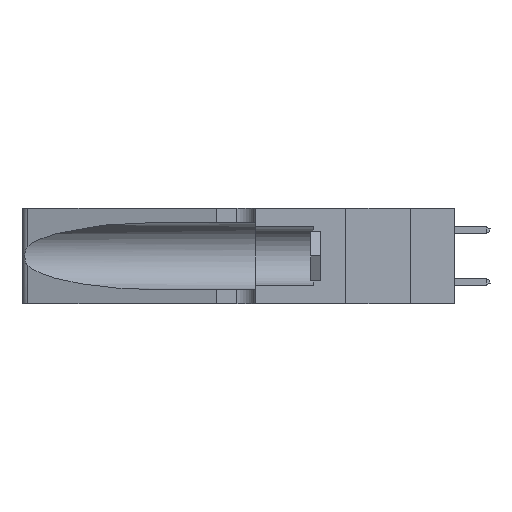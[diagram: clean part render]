
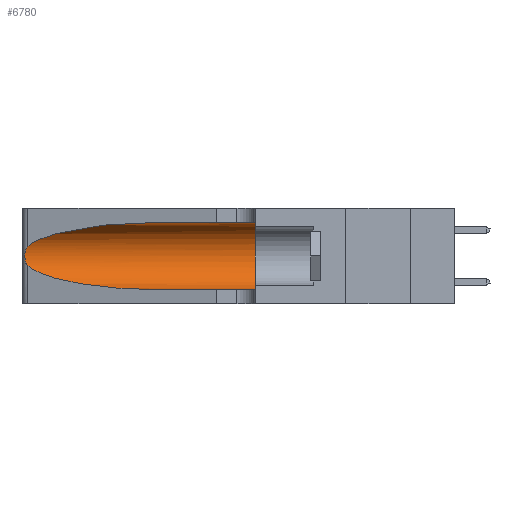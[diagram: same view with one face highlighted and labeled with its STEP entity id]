
A CAD part, left-side view. The second image highlights one B-rep face of the part: STEP entity #6780.
In plain terms, the highlighted cylindrical face has radius 3.308 mm (diameter 6.617 mm), a partial arc.
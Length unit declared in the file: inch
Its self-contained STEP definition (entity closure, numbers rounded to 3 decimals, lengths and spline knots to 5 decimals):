
#3289 = CARTESIAN_POINT ( 'NONE',  ( 0.26075, 1.23896, 0.19203 ) ) ;
#3902 = ORIENTED_EDGE ( 'NONE', *, *, #12680, .F. ) ;
#3939 = CARTESIAN_POINT ( 'NONE',  ( 0.18966, 0.96281, 0.31525 ) ) ;
#4257 = CARTESIAN_POINT ( 'NONE',  ( 0.25487, 1.22718, 0.14631 ) ) ;
#5062 = ORIENTED_EDGE ( 'NONE', *, *, #30417, .T. ) ;
#5416 = DIRECTION ( 'NONE',  ( 0., 1., 0. ) ) ;
#5429 = EDGE_CURVE ( 'NONE', #13423, #27642, #40645, .T. ) ;
#5734 = DIRECTION ( 'NONE',  ( 0., 0., 1. ) ) ;
#6224 = CARTESIAN_POINT ( 'NONE',  ( 0.25487, 1.22718, 0.14631 ) ) ;
#6531 = LINE ( 'NONE', #12979, #15134 ) ;
#6780 = ADVANCED_FACE ( 'NONE', ( #13480 ), #31349, .F. ) ;
#7025 = CARTESIAN_POINT ( 'NONE',  ( 0.25639, 1.23186, 0.15144 ) ) ;
#9495 =( BOUNDED_CURVE ( )  B_SPLINE_CURVE ( 3, ( #40600, #3939, #44308, #36761 ),
 .UNSPECIFIED., .F., .F. ) 
 B_SPLINE_CURVE_WITH_KNOTS ( ( 4, 4 ),
 ( 1.5708, 2.84003 ),
 .UNSPECIFIED. ) 
 CURVE ( )  GEOMETRIC_REPRESENTATION_ITEM ( )  RATIONAL_B_SPLINE_CURVE ( ( 1., 0.87, 0.87, 1. ) ) 
 REPRESENTATION_ITEM ( '' )  );
#10245 = VERTEX_POINT ( 'NONE', #32765 ) ;
#10259 = CARTESIAN_POINT ( 'NONE',  ( 0.25555, 1.22993, 0.14849 ) ) ;
#10776 = AXIS2_PLACEMENT_3D ( 'NONE', #34550, #24108, #42113 ) ;
#12680 = EDGE_CURVE ( 'NONE', #41714, #13423, #20271, .T. ) ;
#12801 = CARTESIAN_POINT ( 'NONE',  ( 0.1305, 0.35, 0.05475 ) ) ;
#12979 = CARTESIAN_POINT ( 'NONE',  ( 0.1305, 1.61858, 0.05475 ) ) ;
#13423 = VERTEX_POINT ( 'NONE', #22677 ) ;
#13480 = FACE_OUTER_BOUND ( 'NONE', #32937, .T. ) ;
#15134 = VECTOR ( 'NONE', #31310, 39.37008 ) ;
#15164 = ORIENTED_EDGE ( 'NONE', *, *, #5429, .F. ) ;
#15608 = AXIS2_PLACEMENT_3D ( 'NONE', #20380, #5416, #5734 ) ;
#15639 = VECTOR ( 'NONE', #41364, 39.37008 ) ;
#17497 = VERTEX_POINT ( 'NONE', #4257 ) ;
#17786 = CARTESIAN_POINT ( 'NONE',  ( 0.26018, 1.23835, 0.19895 ) ) ;
#18111 = CARTESIAN_POINT ( 'NONE',  ( 0.26075, 1.23896, 0.178 ) ) ;
#19822 = ORIENTED_EDGE ( 'NONE', *, *, #21107, .T. ) ;
#20271 = LINE ( 'NONE', #33636, #15639 ) ;
#20380 = CARTESIAN_POINT ( 'NONE',  ( 0.1305, 0.35, 0.185 ) ) ;
#21006 = EDGE_CURVE ( 'NONE', #17497, #45931, #23612, .T. ) ;
#21107 = EDGE_CURVE ( 'NONE', #10245, #17497, #45736, .T. ) ;
#21335 = CARTESIAN_POINT ( 'NONE',  ( 0.26017, 1.23833, 0.17102 ) ) ;
#22677 = CARTESIAN_POINT ( 'NONE',  ( 0.1305, 0.35, 0.31525 ) ) ;
#23612 =( BOUNDED_CURVE ( )  B_SPLINE_CURVE ( 3, ( #6224, #35629, #35780, #24851 ),
 .UNSPECIFIED., .F., .T. ) 
 B_SPLINE_CURVE_WITH_KNOTS ( ( 4, 4 ),
 ( 3.44316, 4.71239 ),
 .UNSPECIFIED. ) 
 CURVE ( )  GEOMETRIC_REPRESENTATION_ITEM ( )  RATIONAL_B_SPLINE_CURVE ( ( 1., 0.87, 0.87, 1. ) ) 
 REPRESENTATION_ITEM ( '' )  );
#24108 = DIRECTION ( 'NONE',  ( 0., -1., 0. ) ) ;
#24851 = CARTESIAN_POINT ( 'NONE',  ( 0.1305, 0.72297, 0.05475 ) ) ;
#25166 = CARTESIAN_POINT ( 'NONE',  ( 0.25787, 1.23484, 0.2124 ) ) ;
#25326 = CARTESIAN_POINT ( 'NONE',  ( 0.25487, 1.22718, 0.22369 ) ) ;
#27642 = VERTEX_POINT ( 'NONE', #12801 ) ;
#28156 = CARTESIAN_POINT ( 'NONE',  ( 0.1305, 0.72297, 0.05475 ) ) ;
#28545 = CARTESIAN_POINT ( 'NONE',  ( 0.25856, 1.23593, 0.16098 ) ) ;
#29025 = CARTESIAN_POINT ( 'NONE',  ( 0.25854, 1.2359, 0.20912 ) ) ;
#29763 = ORIENTED_EDGE ( 'NONE', *, *, #21006, .T. ) ;
#30417 = EDGE_CURVE ( 'NONE', #45931, #27642, #6531, .T. ) ;
#31310 = DIRECTION ( 'NONE',  ( 0., -1., 0. ) ) ;
#31349 = CYLINDRICAL_SURFACE ( 'NONE', #10776, 0.13025 ) ;
#32721 = CARTESIAN_POINT ( 'NONE',  ( 0.25487, 1.22718, 0.14631 ) ) ;
#32765 = CARTESIAN_POINT ( 'NONE',  ( 0.25487, 1.22718, 0.22369 ) ) ;
#32878 = CARTESIAN_POINT ( 'NONE',  ( 0.25555, 1.22994, 0.2215 ) ) ;
#32937 = EDGE_LOOP ( 'NONE', ( #46050, #19822, #29763, #5062, #15164, #3902 ) ) ;
#33636 = CARTESIAN_POINT ( 'NONE',  ( 0.1305, 1.61858, 0.31525 ) ) ;
#34339 = EDGE_CURVE ( 'NONE', #41714, #10245, #9495, .T. ) ;
#34550 = CARTESIAN_POINT ( 'NONE',  ( 0.1305, 1.61858, 0.185 ) ) ;
#35629 = CARTESIAN_POINT ( 'NONE',  ( 0.2373, 1.15595, 0.08982 ) ) ;
#35780 = CARTESIAN_POINT ( 'NONE',  ( 0.18966, 0.96281, 0.05475 ) ) ;
#36761 = CARTESIAN_POINT ( 'NONE',  ( 0.25487, 1.22718, 0.22369 ) ) ;
#40284 = CARTESIAN_POINT ( 'NONE',  ( 0.25789, 1.23486, 0.15765 ) ) ;
#40600 = CARTESIAN_POINT ( 'NONE',  ( 0.1305, 0.72297, 0.31525 ) ) ;
#40645 = CIRCLE ( 'NONE', #15608, 0.13025 ) ;
#41364 = DIRECTION ( 'NONE',  ( 0., -1., 0. ) ) ;
#41714 = VERTEX_POINT ( 'NONE', #46935 ) ;
#42113 = DIRECTION ( 'NONE',  ( 0., 0., -1. ) ) ;
#43978 = CARTESIAN_POINT ( 'NONE',  ( 0.25639, 1.23184, 0.21858 ) ) ;
#44308 = CARTESIAN_POINT ( 'NONE',  ( 0.2373, 1.15595, 0.28018 ) ) ;
#45736 = B_SPLINE_CURVE_WITH_KNOTS ( 'NONE', 3,
 ( #25326, #32878, #43978, #25166, #29025, #17786, #3289, #18111, #21335, #28545, #40284, #7025, #10259, #32721 ),
 .UNSPECIFIED., .F., .F.,
 ( 4, 2, 2, 2, 2, 2, 4 ),
 ( 0., 0.00027, 0.00053, 0.00107, 0.0016, 0.00187, 0.00214 ),
 .UNSPECIFIED. ) ;
#45931 = VERTEX_POINT ( 'NONE', #28156 ) ;
#46050 = ORIENTED_EDGE ( 'NONE', *, *, #34339, .T. ) ;
#46935 = CARTESIAN_POINT ( 'NONE',  ( 0.1305, 0.72297, 0.31525 ) ) ;
